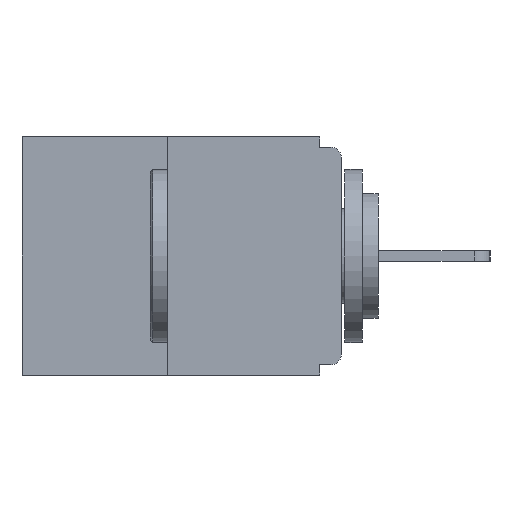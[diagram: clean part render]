
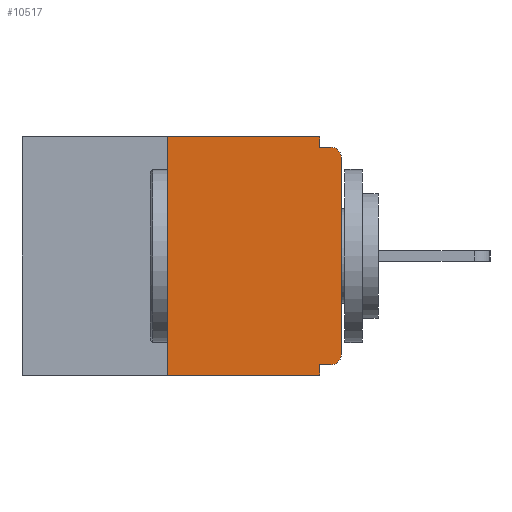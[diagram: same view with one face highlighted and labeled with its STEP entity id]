
A CAD part, left-side view. The second image highlights one B-rep face of the part: STEP entity #10517.
In plain terms, the highlighted planar face has unit normal (-1, 0, 0).
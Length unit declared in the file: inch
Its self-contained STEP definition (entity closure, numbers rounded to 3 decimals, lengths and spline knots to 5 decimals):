
#397 = CARTESIAN_POINT ( 'NONE',  ( 0., 0.031, -0.343 ) ) ;
#505 = ORIENTED_EDGE ( 'NONE', *, *, #22507, .F. ) ;
#523 = DIRECTION ( 'NONE',  ( 0., 0., -1. ) ) ;
#818 = DIRECTION ( 'NONE',  ( 0., -1., 0. ) ) ;
#1889 = EDGE_CURVE ( 'NONE', #22987, #8047, #17278, .T. ) ;
#1957 = CARTESIAN_POINT ( 'NONE',  ( 0., 0., -0.328 ) ) ;
#2281 = AXIS2_PLACEMENT_3D ( 'NONE', #19559, #19431, #21837 ) ;
#2327 = VECTOR ( 'NONE', #11929, 39.37008 ) ;
#2687 = VERTEX_POINT ( 'NONE', #17090 ) ;
#3163 = PLANE ( 'NONE',  #11399 ) ;
#3507 = ORIENTED_EDGE ( 'NONE', *, *, #22622, .F. ) ;
#4200 = CARTESIAN_POINT ( 'NONE',  ( 0., 0.25, 0. ) ) ;
#4267 = CIRCLE ( 'NONE', #2281, 0.015 ) ;
#4725 = CARTESIAN_POINT ( 'NONE',  ( 0., 0.031, -0.343 ) ) ;
#5129 = ORIENTED_EDGE ( 'NONE', *, *, #5139, .F. ) ;
#5139 = EDGE_CURVE ( 'NONE', #2687, #19640, #14812, .T. ) ;
#5249 = VECTOR ( 'NONE', #7701, 39.37008 ) ;
#5347 = DIRECTION ( 'NONE',  ( 0., -1., 0. ) ) ;
#5412 = DIRECTION ( 'NONE',  ( 0., 0., -1. ) ) ;
#5441 = EDGE_CURVE ( 'NONE', #19640, #18557, #11798, .T. ) ;
#5499 = CARTESIAN_POINT ( 'NONE',  ( 0., 0.46, -0.343 ) ) ;
#5718 = CARTESIAN_POINT ( 'NONE',  ( 0., 0.031, -0.328 ) ) ;
#7001 = ORIENTED_EDGE ( 'NONE', *, *, #7046, .T. ) ;
#7046 = EDGE_CURVE ( 'NONE', #7563, #22987, #4267, .T. ) ;
#7131 = CARTESIAN_POINT ( 'NONE',  ( 0., 0.015, -0.03 ) ) ;
#7563 = VERTEX_POINT ( 'NONE', #13490 ) ;
#7701 = DIRECTION ( 'NONE',  ( 0., 0., 1. ) ) ;
#8047 = VERTEX_POINT ( 'NONE', #19625 ) ;
#8133 = CIRCLE ( 'NONE', #16981, 0.015 ) ;
#8234 = FACE_OUTER_BOUND ( 'NONE', #11245, .T. ) ;
#8239 = CARTESIAN_POINT ( 'NONE',  ( 0., 0., -0.313 ) ) ;
#8303 = VERTEX_POINT ( 'NONE', #4725 ) ;
#8536 = CARTESIAN_POINT ( 'NONE',  ( 0., 0.46, 0. ) ) ;
#8586 = VERTEX_POINT ( 'NONE', #5718 ) ;
#8922 = VECTOR ( 'NONE', #818, 39.37008 ) ;
#9124 = VECTOR ( 'NONE', #19368, 39.37008 ) ;
#9272 = CARTESIAN_POINT ( 'NONE',  ( 0., 0., 0. ) ) ;
#9595 = VECTOR ( 'NONE', #9676, 39.37008 ) ;
#9676 = DIRECTION ( 'NONE',  ( 0., 1., 0. ) ) ;
#9704 = EDGE_CURVE ( 'NONE', #18557, #22486, #11066, .T. ) ;
#9819 = ORIENTED_EDGE ( 'NONE', *, *, #9704, .F. ) ;
#10278 = CARTESIAN_POINT ( 'NONE',  ( 0., 0.031, 0. ) ) ;
#10517 = ADVANCED_FACE ( 'NONE', ( #8234 ), #3163, .F. ) ;
#11066 = LINE ( 'NONE', #15062, #12405 ) ;
#11245 = EDGE_LOOP ( 'NONE', ( #5129, #3507, #12502, #16714, #505, #7001, #16939, #11617, #9819, #11806 ) ) ;
#11399 = AXIS2_PLACEMENT_3D ( 'NONE', #22834, #24352, #5412 ) ;
#11617 = ORIENTED_EDGE ( 'NONE', *, *, #14723, .T. ) ;
#11798 = LINE ( 'NONE', #10278, #24241 ) ;
#11806 = ORIENTED_EDGE ( 'NONE', *, *, #5441, .F. ) ;
#11929 = DIRECTION ( 'NONE',  ( 0., 0., 1. ) ) ;
#12405 = VECTOR ( 'NONE', #5347, 39.37008 ) ;
#12502 = ORIENTED_EDGE ( 'NONE', *, *, #19565, .T. ) ;
#13490 = CARTESIAN_POINT ( 'NONE',  ( 0., 0.015, -0.328 ) ) ;
#14723 = EDGE_CURVE ( 'NONE', #8047, #22486, #8133, .T. ) ;
#14789 = EDGE_CURVE ( 'NONE', #8586, #8303, #15651, .T. ) ;
#14812 = LINE ( 'NONE', #8536, #8922 ) ;
#15062 = CARTESIAN_POINT ( 'NONE',  ( 0., 0., -0.015 ) ) ;
#15651 = LINE ( 'NONE', #397, #22613 ) ;
#16710 = DIRECTION ( 'NONE',  ( -1., 0., 0. ) ) ;
#16714 = ORIENTED_EDGE ( 'NONE', *, *, #14789, .F. ) ;
#16939 = ORIENTED_EDGE ( 'NONE', *, *, #1889, .T. ) ;
#16981 = AXIS2_PLACEMENT_3D ( 'NONE', #7131, #16710, #24405 ) ;
#17090 = CARTESIAN_POINT ( 'NONE',  ( 0., 0.25, 0. ) ) ;
#17278 = LINE ( 'NONE', #9272, #5249 ) ;
#17581 = DIRECTION ( 'NONE',  ( 0., 0., -1. ) ) ;
#18557 = VERTEX_POINT ( 'NONE', #22515 ) ;
#18877 = CARTESIAN_POINT ( 'NONE',  ( 0., 0.031, 0. ) ) ;
#19368 = DIRECTION ( 'NONE',  ( 0., -1., 0. ) ) ;
#19431 = DIRECTION ( 'NONE',  ( -1., 0., 0. ) ) ;
#19559 = CARTESIAN_POINT ( 'NONE',  ( 0., 0.015, -0.313 ) ) ;
#19565 = EDGE_CURVE ( 'NONE', #21516, #8303, #22795, .T. ) ;
#19625 = CARTESIAN_POINT ( 'NONE',  ( 0., 0., -0.03 ) ) ;
#19640 = VERTEX_POINT ( 'NONE', #18877 ) ;
#21379 = LINE ( 'NONE', #1957, #9595 ) ;
#21505 = LINE ( 'NONE', #4200, #2327 ) ;
#21516 = VERTEX_POINT ( 'NONE', #24018 ) ;
#21837 = DIRECTION ( 'NONE',  ( 0., 0., -1. ) ) ;
#22486 = VERTEX_POINT ( 'NONE', #23404 ) ;
#22507 = EDGE_CURVE ( 'NONE', #7563, #8586, #21379, .T. ) ;
#22515 = CARTESIAN_POINT ( 'NONE',  ( 0., 0.031, -0.015 ) ) ;
#22613 = VECTOR ( 'NONE', #523, 39.37008 ) ;
#22622 = EDGE_CURVE ( 'NONE', #21516, #2687, #21505, .T. ) ;
#22795 = LINE ( 'NONE', #5499, #9124 ) ;
#22834 = CARTESIAN_POINT ( 'NONE',  ( 0., 0.46, 0. ) ) ;
#22987 = VERTEX_POINT ( 'NONE', #8239 ) ;
#23404 = CARTESIAN_POINT ( 'NONE',  ( 0., 0.015, -0.015 ) ) ;
#24018 = CARTESIAN_POINT ( 'NONE',  ( 0., 0.25, -0.343 ) ) ;
#24241 = VECTOR ( 'NONE', #17581, 39.37008 ) ;
#24352 = DIRECTION ( 'NONE',  ( 1., 0., 0. ) ) ;
#24405 = DIRECTION ( 'NONE',  ( 0., 0., -1. ) ) ;
